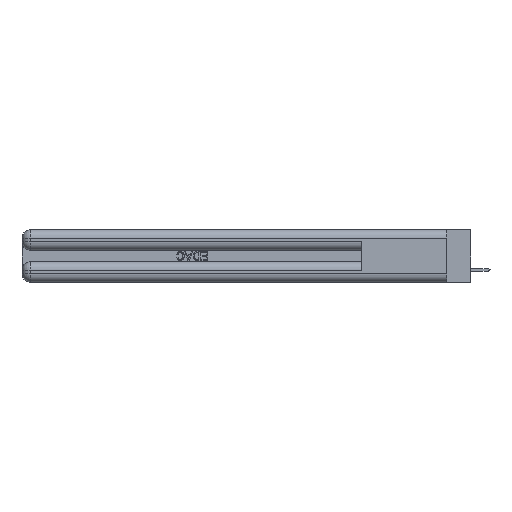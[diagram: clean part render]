
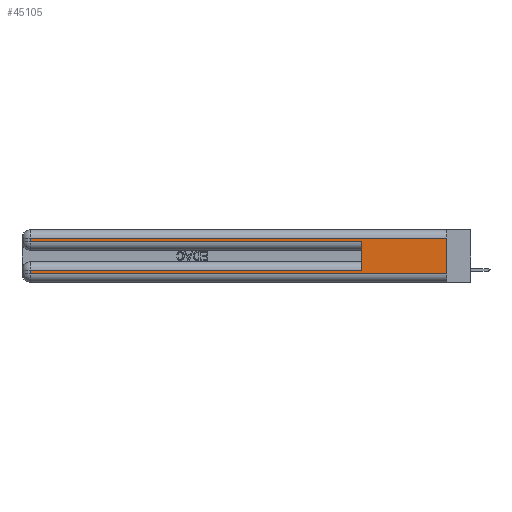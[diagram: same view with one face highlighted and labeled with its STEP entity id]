
A CAD part, left-side view. The second image highlights one B-rep face of the part: STEP entity #45105.
In plain terms, the highlighted planar face has unit normal (-1, 0, 0).
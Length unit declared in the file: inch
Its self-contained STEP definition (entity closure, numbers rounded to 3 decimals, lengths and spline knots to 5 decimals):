
#737 = CARTESIAN_POINT ( 'NONE',  ( 0., 2.94, 0.285 ) ) ;
#2208 = CARTESIAN_POINT ( 'NONE',  ( 0., 0.6, 0.145 ) ) ;
#2279 = VERTEX_POINT ( 'NONE', #44294 ) ;
#4182 = CARTESIAN_POINT ( 'NONE',  ( 0., 2.94, 0.37 ) ) ;
#4426 = ORIENTED_EDGE ( 'NONE', *, *, #15503, .T. ) ;
#5752 = ORIENTED_EDGE ( 'NONE', *, *, #26783, .T. ) ;
#6191 = ORIENTED_EDGE ( 'NONE', *, *, #8092, .F. ) ;
#6541 = DIRECTION ( 'NONE',  ( 0., -1., 0. ) ) ;
#8092 = EDGE_CURVE ( 'NONE', #40044, #33389, #45931, .T. ) ;
#9016 = PLANE ( 'NONE',  #28037 ) ;
#9161 = LINE ( 'NONE', #12947, #27930 ) ;
#10121 = LINE ( 'NONE', #24603, #44981 ) ;
#10520 = LINE ( 'NONE', #2208, #11128 ) ;
#11128 = VECTOR ( 'NONE', #27635, 39.37008 ) ;
#11446 = CARTESIAN_POINT ( 'NONE',  ( 0., 0., 0.085 ) ) ;
#11474 = LINE ( 'NONE', #21940, #30676 ) ;
#11857 = DIRECTION ( 'NONE',  ( 0., 0., -1. ) ) ;
#12326 = VERTEX_POINT ( 'NONE', #14963 ) ;
#12575 = CARTESIAN_POINT ( 'NONE',  ( 0., 0., 0.37 ) ) ;
#12769 = DIRECTION ( 'NONE',  ( 0., 0., -1. ) ) ;
#12947 = CARTESIAN_POINT ( 'NONE',  ( 0., 0., 0.31 ) ) ;
#14963 = CARTESIAN_POINT ( 'NONE',  ( 0., 2.94, 0.31 ) ) ;
#15503 = EDGE_CURVE ( 'NONE', #18888, #17736, #11474, .T. ) ;
#15919 = ORIENTED_EDGE ( 'NONE', *, *, #16365, .T. ) ;
#16092 = VECTOR ( 'NONE', #12769, 39.37008 ) ;
#16363 = DIRECTION ( 'NONE',  ( 1., 0., 0. ) ) ;
#16365 = EDGE_CURVE ( 'NONE', #17736, #33389, #10121, .T. ) ;
#17072 = EDGE_CURVE ( 'NONE', #19213, #2279, #30907, .T. ) ;
#17208 = EDGE_LOOP ( 'NONE', ( #6191, #22768, #5752, #46871, #46527, #36977, #4426, #15919 ) ) ;
#17736 = VERTEX_POINT ( 'NONE', #32960 ) ;
#18210 = DIRECTION ( 'NONE',  ( 0., 0., -1. ) ) ;
#18382 = CARTESIAN_POINT ( 'NONE',  ( 0., 2.94, 0.085 ) ) ;
#18888 = VERTEX_POINT ( 'NONE', #18382 ) ;
#18893 = CARTESIAN_POINT ( 'NONE',  ( 0., 0., 0.31 ) ) ;
#19046 = DIRECTION ( 'NONE',  ( 0., 1., 0. ) ) ;
#19213 = VERTEX_POINT ( 'NONE', #737 ) ;
#21940 = CARTESIAN_POINT ( 'NONE',  ( 0., 2.94, 0.37 ) ) ;
#22768 = ORIENTED_EDGE ( 'NONE', *, *, #23254, .T. ) ;
#23254 = EDGE_CURVE ( 'NONE', #40044, #12326, #9161, .T. ) ;
#23545 = VECTOR ( 'NONE', #19046, 39.37008 ) ;
#23691 = VECTOR ( 'NONE', #18210, 39.37008 ) ;
#24097 = DIRECTION ( 'NONE',  ( 0., 1., 0. ) ) ;
#24603 = CARTESIAN_POINT ( 'NONE',  ( 0., 0., 0.06 ) ) ;
#25293 = EDGE_CURVE ( 'NONE', #46049, #18888, #43916, .T. ) ;
#26783 = EDGE_CURVE ( 'NONE', #12326, #19213, #36200, .T. ) ;
#27635 = DIRECTION ( 'NONE',  ( 0., 0., 1. ) ) ;
#27930 = VECTOR ( 'NONE', #24097, 39.37008 ) ;
#28037 = AXIS2_PLACEMENT_3D ( 'NONE', #12575, #16363, #11857 ) ;
#29507 = DIRECTION ( 'NONE',  ( 0., 0., -1. ) ) ;
#30676 = VECTOR ( 'NONE', #29507, 39.37008 ) ;
#30907 = LINE ( 'NONE', #45354, #46530 ) ;
#31266 = CARTESIAN_POINT ( 'NONE',  ( 0., 0., 0.37 ) ) ;
#32960 = CARTESIAN_POINT ( 'NONE',  ( 0., 2.94, 0.06 ) ) ;
#33389 = VERTEX_POINT ( 'NONE', #37894 ) ;
#34591 = FACE_OUTER_BOUND ( 'NONE', #17208, .T. ) ;
#36200 = LINE ( 'NONE', #4182, #23691 ) ;
#36977 = ORIENTED_EDGE ( 'NONE', *, *, #25293, .T. ) ;
#37305 = DIRECTION ( 'NONE',  ( 0., -1., 0. ) ) ;
#37894 = CARTESIAN_POINT ( 'NONE',  ( 0., 0., 0.06 ) ) ;
#39064 = EDGE_CURVE ( 'NONE', #46049, #2279, #10520, .T. ) ;
#40044 = VERTEX_POINT ( 'NONE', #18893 ) ;
#40439 = CARTESIAN_POINT ( 'NONE',  ( 0., 0.6, 0.085 ) ) ;
#43916 = LINE ( 'NONE', #11446, #23545 ) ;
#44294 = CARTESIAN_POINT ( 'NONE',  ( 0., 0.6, 0.285 ) ) ;
#44981 = VECTOR ( 'NONE', #6541, 39.37008 ) ;
#45105 = ADVANCED_FACE ( 'NONE', ( #34591 ), #9016, .F. ) ;
#45354 = CARTESIAN_POINT ( 'NONE',  ( 0., 0., 0.285 ) ) ;
#45931 = LINE ( 'NONE', #31266, #16092 ) ;
#46049 = VERTEX_POINT ( 'NONE', #40439 ) ;
#46527 = ORIENTED_EDGE ( 'NONE', *, *, #39064, .F. ) ;
#46530 = VECTOR ( 'NONE', #37305, 39.37008 ) ;
#46871 = ORIENTED_EDGE ( 'NONE', *, *, #17072, .T. ) ;
